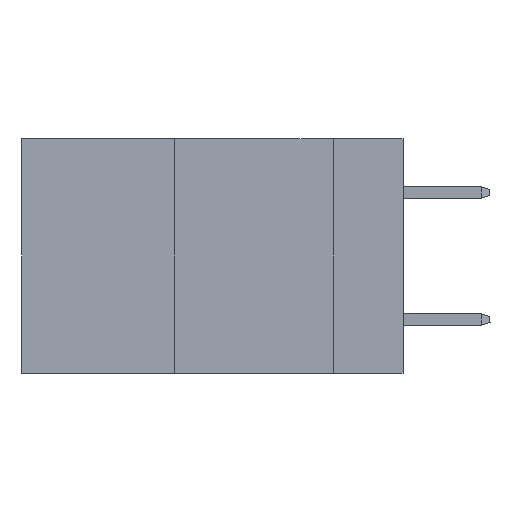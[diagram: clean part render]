
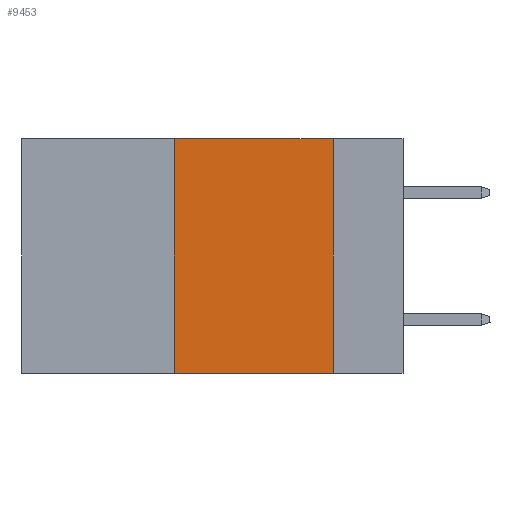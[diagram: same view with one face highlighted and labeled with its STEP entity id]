
A CAD part, left-side view. The second image highlights one B-rep face of the part: STEP entity #9453.
In plain terms, the highlighted planar face has unit normal (-1, 0, 0).
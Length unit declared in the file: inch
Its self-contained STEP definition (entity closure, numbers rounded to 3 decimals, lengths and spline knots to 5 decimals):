
#27 = CARTESIAN_POINT ( 'NONE',  ( 0., 0.36, 0. ) ) ;
#160 = DIRECTION ( 'NONE',  ( 1., 0., 0. ) ) ;
#198 = VERTEX_POINT ( 'NONE', #12140 ) ;
#1030 = EDGE_CURVE ( 'NONE', #8919, #12173, #8545, .T. ) ;
#1147 = LINE ( 'NONE', #2797, #19879 ) ;
#2406 = CARTESIAN_POINT ( 'NONE',  ( 0., 0.6, 0. ) ) ;
#2797 = CARTESIAN_POINT ( 'NONE',  ( 0., 0.6, -0.37 ) ) ;
#3341 = CARTESIAN_POINT ( 'NONE',  ( 0., 0.36, 0. ) ) ;
#3818 = DIRECTION ( 'NONE',  ( 0., -1., 0. ) ) ;
#4174 = EDGE_CURVE ( 'NONE', #12173, #9268, #7095, .T. ) ;
#6896 = VECTOR ( 'NONE', #3818, 39.37008 ) ;
#7095 = LINE ( 'NONE', #10450, #6896 ) ;
#8190 = EDGE_LOOP ( 'NONE', ( #10830, #19857, #15887, #14357 ) ) ;
#8545 = LINE ( 'NONE', #27, #20856 ) ;
#8919 = VERTEX_POINT ( 'NONE', #16825 ) ;
#9166 = DIRECTION ( 'NONE',  ( 0., 0., -1. ) ) ;
#9265 = PLANE ( 'NONE',  #10841 ) ;
#9268 = VERTEX_POINT ( 'NONE', #15059 ) ;
#9453 = ADVANCED_FACE ( 'NONE', ( #12012 ), #9265, .F. ) ;
#10450 = CARTESIAN_POINT ( 'NONE',  ( 0., 0.6, 0. ) ) ;
#10830 = ORIENTED_EDGE ( 'NONE', *, *, #20887, .F. ) ;
#10841 = AXIS2_PLACEMENT_3D ( 'NONE', #2406, #160, #13439 ) ;
#12012 = FACE_OUTER_BOUND ( 'NONE', #8190, .T. ) ;
#12140 = CARTESIAN_POINT ( 'NONE',  ( 0., 0.11, -0.37 ) ) ;
#12173 = VERTEX_POINT ( 'NONE', #3341 ) ;
#12753 = CARTESIAN_POINT ( 'NONE',  ( 0., 0.11, 0. ) ) ;
#13439 = DIRECTION ( 'NONE',  ( 0., 0., -1. ) ) ;
#14357 = ORIENTED_EDGE ( 'NONE', *, *, #17567, .T. ) ;
#14484 = LINE ( 'NONE', #12753, #14784 ) ;
#14784 = VECTOR ( 'NONE', #9166, 39.37008 ) ;
#15059 = CARTESIAN_POINT ( 'NONE',  ( 0., 0.11, 0. ) ) ;
#15148 = DIRECTION ( 'NONE',  ( 0., 0., 1. ) ) ;
#15887 = ORIENTED_EDGE ( 'NONE', *, *, #1030, .F. ) ;
#16825 = CARTESIAN_POINT ( 'NONE',  ( 0., 0.36, -0.37 ) ) ;
#17567 = EDGE_CURVE ( 'NONE', #8919, #198, #1147, .T. ) ;
#17579 = DIRECTION ( 'NONE',  ( 0., -1., 0. ) ) ;
#19857 = ORIENTED_EDGE ( 'NONE', *, *, #4174, .F. ) ;
#19879 = VECTOR ( 'NONE', #17579, 39.37008 ) ;
#20856 = VECTOR ( 'NONE', #15148, 39.37008 ) ;
#20887 = EDGE_CURVE ( 'NONE', #9268, #198, #14484, .T. ) ;
